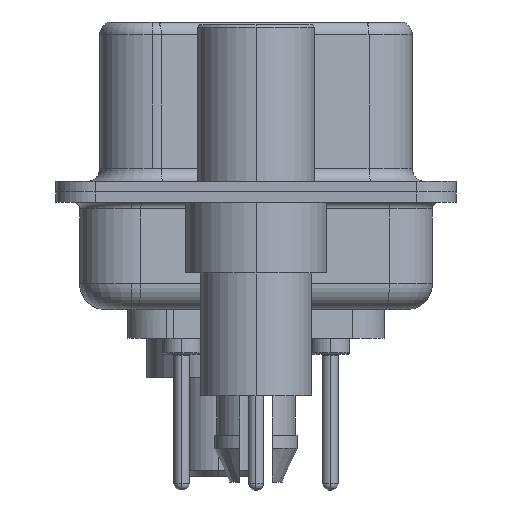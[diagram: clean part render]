
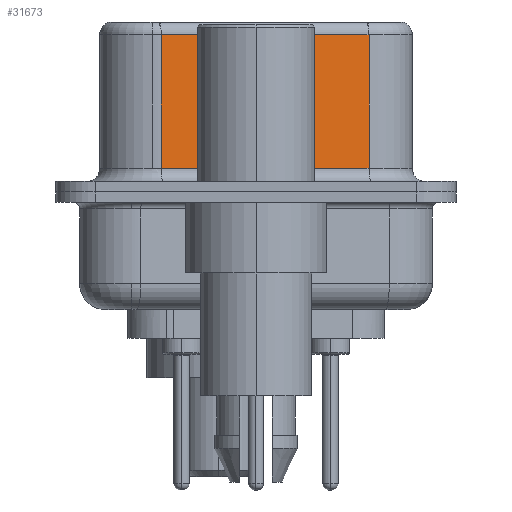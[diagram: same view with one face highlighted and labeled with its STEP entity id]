
A CAD part, left-side view. The second image highlights one B-rep face of the part: STEP entity #31673.
In plain terms, the highlighted planar face has unit normal (-0.985, -0.174, 0).
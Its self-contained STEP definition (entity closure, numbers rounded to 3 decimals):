
#549 = VERTEX_POINT ( 'NONE', #1702 ) ;
#1702 = CARTESIAN_POINT ( 'NONE',  ( 3.73, 3.628, 6.02 ) ) ;
#1988 = VERTEX_POINT ( 'NONE', #4750 ) ;
#2035 = VECTOR ( 'NONE', #13047, 1000. ) ;
#2336 = EDGE_LOOP ( 'NONE', ( #31067, #25299, #11500, #9042 ) ) ;
#3583 = DIRECTION ( 'NONE',  ( -0.174, 0.985, 0. ) ) ;
#4750 = CARTESIAN_POINT ( 'NONE',  ( 5.132, -4.322, 0.9 ) ) ;
#8655 = VECTOR ( 'NONE', #27810, 1000. ) ;
#9042 = ORIENTED_EDGE ( 'NONE', *, *, #9257, .T. ) ;
#9257 = EDGE_CURVE ( 'NONE', #22186, #1988, #14998, .T. ) ;
#9537 = VERTEX_POINT ( 'NONE', #26188 ) ;
#9661 = FACE_OUTER_BOUND ( 'NONE', #2336, .T. ) ;
#10017 = LINE ( 'NONE', #20822, #15702 ) ;
#10126 = LINE ( 'NONE', #17840, #2035 ) ;
#10191 = LINE ( 'NONE', #15522, #8655 ) ;
#11165 = DIRECTION ( 'NONE',  ( 0.174, -0.985, 0. ) ) ;
#11500 = ORIENTED_EDGE ( 'NONE', *, *, #21203, .T. ) ;
#11841 = AXIS2_PLACEMENT_3D ( 'NONE', #25464, #18250, #3583 ) ;
#13047 = DIRECTION ( 'NONE',  ( 0., 0., -1. ) ) ;
#13647 = DIRECTION ( 'NONE',  ( -0.174, 0.985, 0. ) ) ;
#14998 = LINE ( 'NONE', #28339, #20782 ) ;
#15522 = CARTESIAN_POINT ( 'NONE',  ( 5.132, -4.322, 6.52 ) ) ;
#15702 = VECTOR ( 'NONE', #13647, 1000. ) ;
#17840 = CARTESIAN_POINT ( 'NONE',  ( 3.73, 3.628, 6.52 ) ) ;
#18250 = DIRECTION ( 'NONE',  ( 0.985, 0.174, 0. ) ) ;
#20782 = VECTOR ( 'NONE', #11165, 1000. ) ;
#20822 = CARTESIAN_POINT ( 'NONE',  ( 5.132, -4.322, 6.02 ) ) ;
#21203 = EDGE_CURVE ( 'NONE', #549, #22186, #10126, .T. ) ;
#22186 = VERTEX_POINT ( 'NONE', #25856 ) ;
#24187 = EDGE_CURVE ( 'NONE', #9537, #549, #10017, .T. ) ;
#25299 = ORIENTED_EDGE ( 'NONE', *, *, #24187, .T. ) ;
#25464 = CARTESIAN_POINT ( 'NONE',  ( 5.132, -4.322, 6.52 ) ) ;
#25856 = CARTESIAN_POINT ( 'NONE',  ( 3.73, 3.628, 0.9 ) ) ;
#26188 = CARTESIAN_POINT ( 'NONE',  ( 5.132, -4.322, 6.02 ) ) ;
#27810 = DIRECTION ( 'NONE',  ( 0., 0., -1. ) ) ;
#27926 = EDGE_CURVE ( 'NONE', #9537, #1988, #10191, .T. ) ;
#28339 = CARTESIAN_POINT ( 'NONE',  ( 5.132, -4.322, 0.9 ) ) ;
#30576 = PLANE ( 'NONE',  #11841 ) ;
#31067 = ORIENTED_EDGE ( 'NONE', *, *, #27926, .F. ) ;
#31673 = ADVANCED_FACE ( 'NONE', ( #9661 ), #30576, .F. ) ;
